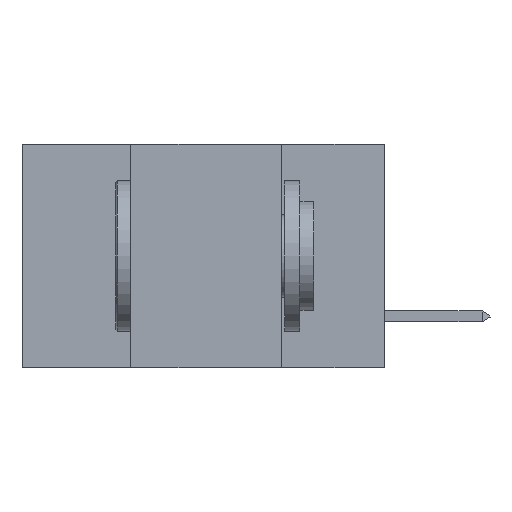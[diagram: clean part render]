
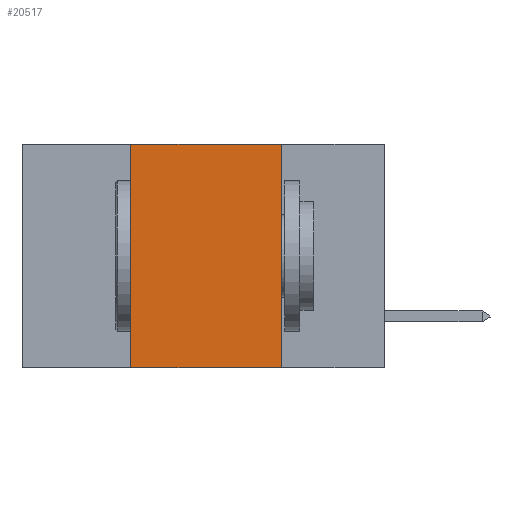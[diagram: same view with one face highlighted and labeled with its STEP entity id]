
A CAD part, left-side view. The second image highlights one B-rep face of the part: STEP entity #20517.
In plain terms, the highlighted planar face has unit normal (-1, 0, 0).
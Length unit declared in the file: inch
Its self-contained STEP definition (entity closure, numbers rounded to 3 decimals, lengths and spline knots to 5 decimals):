
#2263 = EDGE_CURVE ( 'NONE', #3577, #33849, #21012, .T. ) ;
#2676 = CARTESIAN_POINT ( 'NONE',  ( 0., 0.42, 0. ) ) ;
#2951 = ORIENTED_EDGE ( 'NONE', *, *, #32764, .F. ) ;
#3220 = CARTESIAN_POINT ( 'NONE',  ( 0., 0.6, 0. ) ) ;
#3577 = VERTEX_POINT ( 'NONE', #19811 ) ;
#4367 = CARTESIAN_POINT ( 'NONE',  ( 0., 0.6, -0.37 ) ) ;
#5282 = EDGE_LOOP ( 'NONE', ( #46819, #2951, #33420, #12774 ) ) ;
#7033 = EDGE_CURVE ( 'NONE', #3577, #10554, #46099, .T. ) ;
#8405 = DIRECTION ( 'NONE',  ( 0., 0., -1. ) ) ;
#10257 = LINE ( 'NONE', #47075, #39741 ) ;
#10554 = VERTEX_POINT ( 'NONE', #2676 ) ;
#12774 = ORIENTED_EDGE ( 'NONE', *, *, #2263, .T. ) ;
#16265 = CARTESIAN_POINT ( 'NONE',  ( 0., 0.6, 0. ) ) ;
#17397 = VECTOR ( 'NONE', #23482, 39.37008 ) ;
#19242 = VECTOR ( 'NONE', #22830, 39.37008 ) ;
#19811 = CARTESIAN_POINT ( 'NONE',  ( 0., 0.42, -0.37 ) ) ;
#20517 = ADVANCED_FACE ( 'NONE', ( #22801 ), #35626, .F. ) ;
#21012 = LINE ( 'NONE', #4367, #17397 ) ;
#22801 = FACE_OUTER_BOUND ( 'NONE', #5282, .T. ) ;
#22830 = DIRECTION ( 'NONE',  ( 0., -1., 0. ) ) ;
#23482 = DIRECTION ( 'NONE',  ( 0., -1., 0. ) ) ;
#26857 = VECTOR ( 'NONE', #38556, 39.37008 ) ;
#27895 = DIRECTION ( 'NONE',  ( 1., 0., 0. ) ) ;
#27992 = VERTEX_POINT ( 'NONE', #47059 ) ;
#32764 = EDGE_CURVE ( 'NONE', #10554, #27992, #42191, .T. ) ;
#33130 = EDGE_CURVE ( 'NONE', #27992, #33849, #10257, .T. ) ;
#33420 = ORIENTED_EDGE ( 'NONE', *, *, #7033, .F. ) ;
#33849 = VERTEX_POINT ( 'NONE', #44952 ) ;
#34520 = CARTESIAN_POINT ( 'NONE',  ( 0., 0.42, 0. ) ) ;
#35626 = PLANE ( 'NONE',  #40283 ) ;
#38556 = DIRECTION ( 'NONE',  ( 0., 0., 1. ) ) ;
#39741 = VECTOR ( 'NONE', #47743, 39.37008 ) ;
#40283 = AXIS2_PLACEMENT_3D ( 'NONE', #16265, #27895, #8405 ) ;
#42191 = LINE ( 'NONE', #3220, #19242 ) ;
#44952 = CARTESIAN_POINT ( 'NONE',  ( 0., 0.17, -0.37 ) ) ;
#46099 = LINE ( 'NONE', #34520, #26857 ) ;
#46819 = ORIENTED_EDGE ( 'NONE', *, *, #33130, .F. ) ;
#47059 = CARTESIAN_POINT ( 'NONE',  ( 0., 0.17, 0. ) ) ;
#47075 = CARTESIAN_POINT ( 'NONE',  ( 0., 0.17, 0. ) ) ;
#47743 = DIRECTION ( 'NONE',  ( 0., 0., -1. ) ) ;
